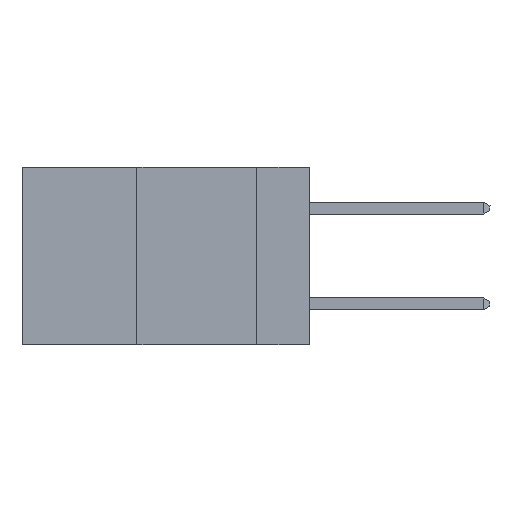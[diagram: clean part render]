
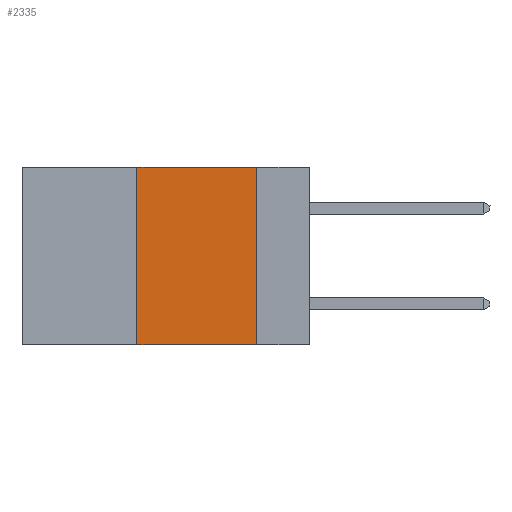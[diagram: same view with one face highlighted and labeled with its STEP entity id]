
A CAD part, left-side view. The second image highlights one B-rep face of the part: STEP entity #2335.
In plain terms, the highlighted planar face has unit normal (-1, 0, 0).
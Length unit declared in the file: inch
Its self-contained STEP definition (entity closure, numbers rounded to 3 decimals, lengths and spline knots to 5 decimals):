
#35 = VERTEX_POINT ( 'NONE', #7791 ) ;
#255 = FACE_OUTER_BOUND ( 'NONE', #2433, .T. ) ;
#367 = ORIENTED_EDGE ( 'NONE', *, *, #2913, .T. ) ;
#750 = VECTOR ( 'NONE', #5500, 39.37008 ) ;
#1360 = LINE ( 'NONE', #1825, #750 ) ;
#1454 = DIRECTION ( 'NONE',  ( 0., 0., 1. ) ) ;
#1825 = CARTESIAN_POINT ( 'NONE',  ( 0., 0.6, 0. ) ) ;
#2335 = ADVANCED_FACE ( 'NONE', ( #255 ), #4980, .F. ) ;
#2433 = EDGE_LOOP ( 'NONE', ( #4336, #6284, #8218, #367 ) ) ;
#2467 = EDGE_CURVE ( 'NONE', #2519, #35, #9076, .T. ) ;
#2519 = VERTEX_POINT ( 'NONE', #7089 ) ;
#2543 = DIRECTION ( 'NONE',  ( 0., 0., -1. ) ) ;
#2716 = VERTEX_POINT ( 'NONE', #7505 ) ;
#2913 = EDGE_CURVE ( 'NONE', #9393, #35, #9702, .T. ) ;
#3937 = DIRECTION ( 'NONE',  ( 1., 0., 0. ) ) ;
#4112 = CARTESIAN_POINT ( 'NONE',  ( 0., 0.36, -0.37 ) ) ;
#4182 = LINE ( 'NONE', #4408, #5886 ) ;
#4336 = ORIENTED_EDGE ( 'NONE', *, *, #2467, .F. ) ;
#4408 = CARTESIAN_POINT ( 'NONE',  ( 0., 0.36, 0. ) ) ;
#4980 = PLANE ( 'NONE',  #9635 ) ;
#5272 = VECTOR ( 'NONE', #8508, 39.37008 ) ;
#5500 = DIRECTION ( 'NONE',  ( 0., -1., 0. ) ) ;
#5792 = CARTESIAN_POINT ( 'NONE',  ( 0., 0.11, 0. ) ) ;
#5886 = VECTOR ( 'NONE', #1454, 39.37008 ) ;
#5954 = VECTOR ( 'NONE', #8484, 39.37008 ) ;
#6284 = ORIENTED_EDGE ( 'NONE', *, *, #8625, .F. ) ;
#7089 = CARTESIAN_POINT ( 'NONE',  ( 0., 0.11, 0. ) ) ;
#7505 = CARTESIAN_POINT ( 'NONE',  ( 0., 0.36, 0. ) ) ;
#7791 = CARTESIAN_POINT ( 'NONE',  ( 0., 0.11, -0.37 ) ) ;
#8218 = ORIENTED_EDGE ( 'NONE', *, *, #8313, .F. ) ;
#8250 = CARTESIAN_POINT ( 'NONE',  ( 0., 0.6, 0. ) ) ;
#8313 = EDGE_CURVE ( 'NONE', #9393, #2716, #4182, .T. ) ;
#8484 = DIRECTION ( 'NONE',  ( 0., -1., 0. ) ) ;
#8508 = DIRECTION ( 'NONE',  ( 0., 0., -1. ) ) ;
#8589 = CARTESIAN_POINT ( 'NONE',  ( 0., 0.6, -0.37 ) ) ;
#8625 = EDGE_CURVE ( 'NONE', #2716, #2519, #1360, .T. ) ;
#9076 = LINE ( 'NONE', #5792, #5272 ) ;
#9393 = VERTEX_POINT ( 'NONE', #4112 ) ;
#9635 = AXIS2_PLACEMENT_3D ( 'NONE', #8250, #3937, #2543 ) ;
#9702 = LINE ( 'NONE', #8589, #5954 ) ;
